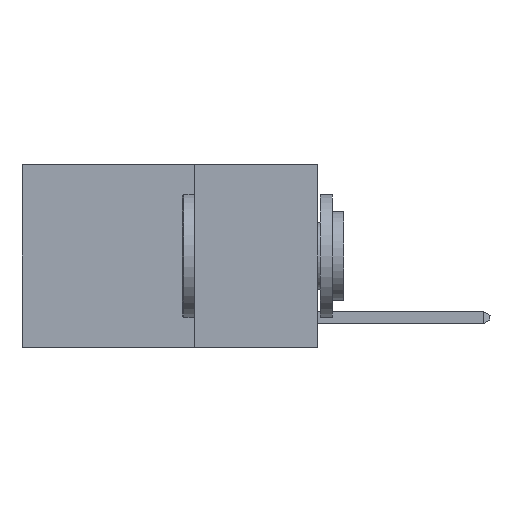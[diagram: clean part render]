
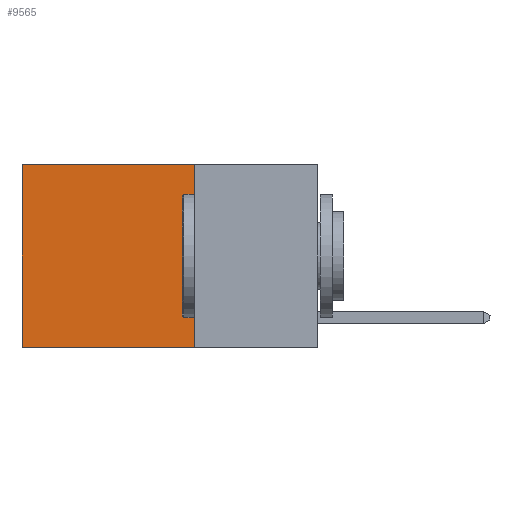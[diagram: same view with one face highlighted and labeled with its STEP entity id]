
A CAD part, left-side view. The second image highlights one B-rep face of the part: STEP entity #9565.
In plain terms, the highlighted planar face has unit normal (-1, 0, 0).
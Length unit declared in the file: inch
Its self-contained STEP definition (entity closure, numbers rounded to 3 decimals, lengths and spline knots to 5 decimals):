
#357 = ORIENTED_EDGE ( 'NONE', *, *, #1302, .F. ) ;
#606 = AXIS2_PLACEMENT_3D ( 'NONE', #26787, #22712, #6893 ) ;
#900 = VECTOR ( 'NONE', #8028, 39.37008 ) ;
#1302 = EDGE_CURVE ( 'NONE', #14206, #21170, #15461, .T. ) ;
#1383 = CARTESIAN_POINT ( 'NONE',  ( 0.2625, 0.25, -0.37 ) ) ;
#1810 = DIRECTION ( 'NONE',  ( 0., 0., -1. ) ) ;
#2236 = ORIENTED_EDGE ( 'NONE', *, *, #16449, .F. ) ;
#2275 = FACE_OUTER_BOUND ( 'NONE', #23050, .T. ) ;
#2598 = EDGE_CURVE ( 'NONE', #8375, #4573, #10968, .T. ) ;
#3358 = CARTESIAN_POINT ( 'NONE',  ( 0.2625, 0.6, -0.37 ) ) ;
#4573 = VERTEX_POINT ( 'NONE', #3358 ) ;
#5015 = PLANE ( 'NONE',  #606 ) ;
#5439 = CARTESIAN_POINT ( 'NONE',  ( 0.2625, 0.6, 0. ) ) ;
#5465 = CARTESIAN_POINT ( 'NONE',  ( 0.2625, 0.25, -0.37 ) ) ;
#6893 = DIRECTION ( 'NONE',  ( 0., 0., -1. ) ) ;
#7653 = ORIENTED_EDGE ( 'NONE', *, *, #19550, .T. ) ;
#8028 = DIRECTION ( 'NONE',  ( 0., 1., 0. ) ) ;
#8182 = CARTESIAN_POINT ( 'NONE',  ( 0.2625, 0.6, 0. ) ) ;
#8375 = VERTEX_POINT ( 'NONE', #5439 ) ;
#9205 = DIRECTION ( 'NONE',  ( 0., 0., -1. ) ) ;
#9565 = ADVANCED_FACE ( 'NONE', ( #2275 ), #5015, .F. ) ;
#10968 = LINE ( 'NONE', #8182, #12851 ) ;
#12851 = VECTOR ( 'NONE', #1810, 39.37008 ) ;
#14206 = VERTEX_POINT ( 'NONE', #28394 ) ;
#15461 = LINE ( 'NONE', #15754, #24314 ) ;
#15754 = CARTESIAN_POINT ( 'NONE',  ( 0.2625, 0.25, 0. ) ) ;
#16449 = EDGE_CURVE ( 'NONE', #21170, #4573, #26014, .T. ) ;
#17233 = VECTOR ( 'NONE', #22622, 39.37008 ) ;
#19550 = EDGE_CURVE ( 'NONE', #14206, #8375, #25379, .T. ) ;
#21170 = VERTEX_POINT ( 'NONE', #5465 ) ;
#22622 = DIRECTION ( 'NONE',  ( 0., 1., 0. ) ) ;
#22712 = DIRECTION ( 'NONE',  ( 1., 0., 0. ) ) ;
#22764 = CARTESIAN_POINT ( 'NONE',  ( 0.2625, 0.25, 0. ) ) ;
#23050 = EDGE_LOOP ( 'NONE', ( #26548, #2236, #357, #7653 ) ) ;
#24314 = VECTOR ( 'NONE', #9205, 39.37008 ) ;
#25379 = LINE ( 'NONE', #22764, #17233 ) ;
#26014 = LINE ( 'NONE', #1383, #900 ) ;
#26548 = ORIENTED_EDGE ( 'NONE', *, *, #2598, .T. ) ;
#26787 = CARTESIAN_POINT ( 'NONE',  ( 0.2625, 0.25, 0. ) ) ;
#28394 = CARTESIAN_POINT ( 'NONE',  ( 0.2625, 0.25, 0. ) ) ;
